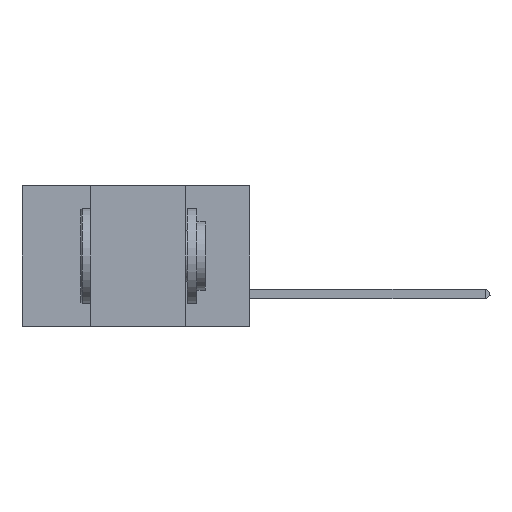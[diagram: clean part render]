
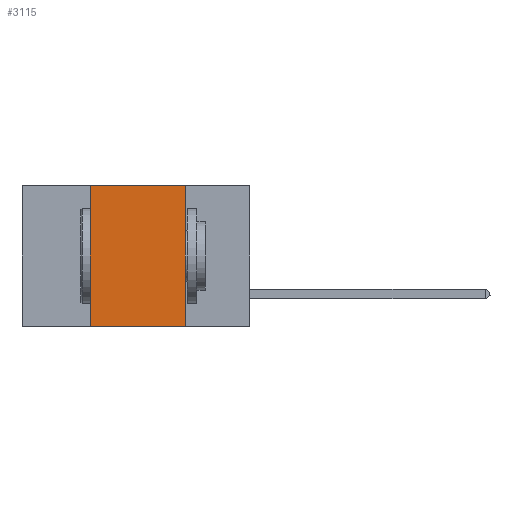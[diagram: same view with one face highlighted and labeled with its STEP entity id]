
A CAD part, left-side view. The second image highlights one B-rep face of the part: STEP entity #3115.
In plain terms, the highlighted planar face has unit normal (-1, 0, 0).
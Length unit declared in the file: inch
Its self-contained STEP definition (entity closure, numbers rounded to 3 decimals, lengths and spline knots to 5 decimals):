
#2928 = ORIENTED_EDGE ( 'NONE', *, *, #23619, .F. ) ;
#3057 = VERTEX_POINT ( 'NONE', #14133 ) ;
#3115 = ADVANCED_FACE ( 'NONE', ( #36109 ), #23601, .F. ) ;
#4437 = EDGE_CURVE ( 'NONE', #10968, #25305, #32813, .T. ) ;
#6908 = CARTESIAN_POINT ( 'NONE',  ( 0., 0.6, 0. ) ) ;
#8453 = CARTESIAN_POINT ( 'NONE',  ( 0., 0.17, 0. ) ) ;
#10286 = DIRECTION ( 'NONE',  ( 1., 0., 0. ) ) ;
#10968 = VERTEX_POINT ( 'NONE', #39024 ) ;
#11637 = VECTOR ( 'NONE', #32185, 39.37008 ) ;
#13714 = AXIS2_PLACEMENT_3D ( 'NONE', #6908, #10286, #34138 ) ;
#13938 = CARTESIAN_POINT ( 'NONE',  ( 0., 0.6, -0.37 ) ) ;
#14133 = CARTESIAN_POINT ( 'NONE',  ( 0., 0.42, 0. ) ) ;
#14630 = LINE ( 'NONE', #31010, #17289 ) ;
#17065 = DIRECTION ( 'NONE',  ( 0., -1., 0. ) ) ;
#17289 = VECTOR ( 'NONE', #41232, 39.37008 ) ;
#18898 = CARTESIAN_POINT ( 'NONE',  ( 0., 0.6, 0. ) ) ;
#21276 = ORIENTED_EDGE ( 'NONE', *, *, #23371, .F. ) ;
#23371 = EDGE_CURVE ( 'NONE', #39778, #25305, #38887, .T. ) ;
#23415 = LINE ( 'NONE', #18898, #11637 ) ;
#23601 = PLANE ( 'NONE',  #13714 ) ;
#23619 = EDGE_CURVE ( 'NONE', #3057, #39778, #23415, .T. ) ;
#24224 = VECTOR ( 'NONE', #17065, 39.37008 ) ;
#25305 = VERTEX_POINT ( 'NONE', #39845 ) ;
#29877 = VECTOR ( 'NONE', #32287, 39.37008 ) ;
#31010 = CARTESIAN_POINT ( 'NONE',  ( 0., 0.42, 0. ) ) ;
#32185 = DIRECTION ( 'NONE',  ( 0., -1., 0. ) ) ;
#32287 = DIRECTION ( 'NONE',  ( 0., 0., -1. ) ) ;
#32577 = EDGE_LOOP ( 'NONE', ( #21276, #2928, #39808, #38853 ) ) ;
#32813 = LINE ( 'NONE', #13938, #24224 ) ;
#33160 = CARTESIAN_POINT ( 'NONE',  ( 0., 0.17, 0. ) ) ;
#34138 = DIRECTION ( 'NONE',  ( 0., 0., -1. ) ) ;
#36109 = FACE_OUTER_BOUND ( 'NONE', #32577, .T. ) ;
#38853 = ORIENTED_EDGE ( 'NONE', *, *, #4437, .T. ) ;
#38887 = LINE ( 'NONE', #33160, #29877 ) ;
#39024 = CARTESIAN_POINT ( 'NONE',  ( 0., 0.42, -0.37 ) ) ;
#39778 = VERTEX_POINT ( 'NONE', #8453 ) ;
#39808 = ORIENTED_EDGE ( 'NONE', *, *, #42771, .F. ) ;
#39845 = CARTESIAN_POINT ( 'NONE',  ( 0., 0.17, -0.37 ) ) ;
#41232 = DIRECTION ( 'NONE',  ( 0., 0., 1. ) ) ;
#42771 = EDGE_CURVE ( 'NONE', #10968, #3057, #14630, .T. ) ;
